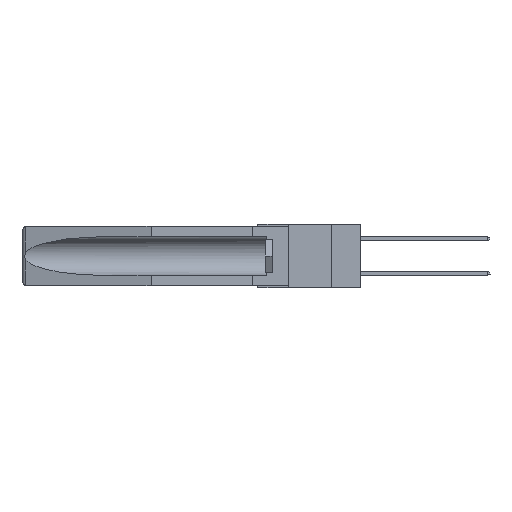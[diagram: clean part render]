
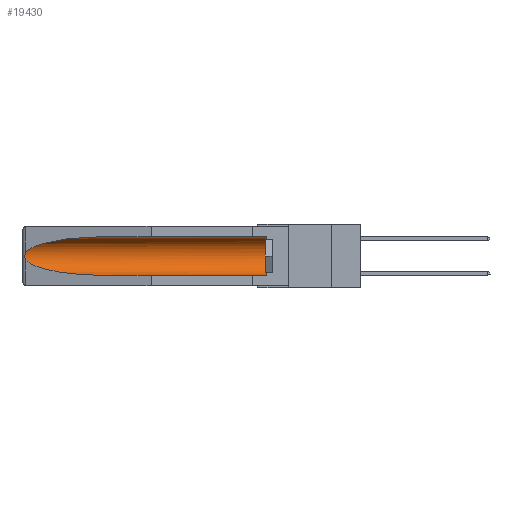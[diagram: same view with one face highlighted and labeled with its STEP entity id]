
A CAD part, left-side view. The second image highlights one B-rep face of the part: STEP entity #19430.
In plain terms, the highlighted cylindrical face has radius 2.857 mm (diameter 5.715 mm), a partial arc.
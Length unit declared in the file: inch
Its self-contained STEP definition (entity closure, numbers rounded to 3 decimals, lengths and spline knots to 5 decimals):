
#130 = CARTESIAN_POINT ( 'NONE',  ( 0.25451, 1.48313, -0.24835 ) ) ;
#312 = EDGE_LOOP ( 'NONE', ( #9508, #18274, #1565, #18513, #764, #6808 ) ) ;
#373 = CARTESIAN_POINT ( 'NONE',  ( 0.2673, 1.53269, -0.17917 ) ) ;
#441 = CARTESIAN_POINT ( 'NONE',  ( 0.2675, 1.53308, -0.16763 ) ) ;
#499 = DIRECTION ( 'NONE',  ( 0., 1., 0. ) ) ;
#579 = EDGE_CURVE ( 'NONE', #10591, #4439, #4516, .T. ) ;
#764 = ORIENTED_EDGE ( 'NONE', *, *, #3685, .T. ) ;
#1401 = CARTESIAN_POINT ( 'NONE',  ( 0.26537, 1.52718, -0.14972 ) ) ;
#1555 = CARTESIAN_POINT ( 'NONE',  ( 0.21114, 1.30732, -0.059 ) ) ;
#1565 = ORIENTED_EDGE ( 'NONE', *, *, #3942, .T. ) ;
#1609 = CARTESIAN_POINT ( 'NONE',  ( 0.21114, 1.30732, -0.284 ) ) ;
#2136 = CARTESIAN_POINT ( 'NONE',  ( 0.26597, 1.5296, -0.19026 ) ) ;
#2745 = DIRECTION ( 'NONE',  ( 0., 0., 1. ) ) ;
#3204 =( BOUNDED_CURVE ( )  B_SPLINE_CURVE ( 3, ( #21183, #1555, #11333, #11249 ),
 .UNSPECIFIED., .F., .F. ) 
 B_SPLINE_CURVE_WITH_KNOTS ( ( 4, 4 ),
 ( 4.71239, 6.08839 ),
 .UNSPECIFIED. ) 
 CURVE ( )  GEOMETRIC_REPRESENTATION_ITEM ( )  RATIONAL_B_SPLINE_CURVE ( ( 1., 0.848, 0.848, 1. ) ) 
 REPRESENTATION_ITEM ( '' )  );
#3685 = EDGE_CURVE ( 'NONE', #10591, #5957, #14403, .T. ) ;
#3721 = EDGE_CURVE ( 'NONE', #5957, #11192, #7472, .T. ) ;
#3915 = B_SPLINE_CURVE_WITH_KNOTS ( 'NONE', 3,
 ( #11846, #15099, #11992, #5355, #441, #16860, #373, #6853, #2136, #18375 ),
 .UNSPECIFIED., .F., .F.,
 ( 4, 2, 2, 2, 4 ),
 ( 0., 0.00029, 0.00058, 0.00087, 0.00117 ),
 .UNSPECIFIED. ) ;
#3942 = EDGE_CURVE ( 'NONE', #12781, #4439, #20276, .T. ) ;
#4372 = CARTESIAN_POINT ( 'NONE',  ( 0.155, 0.126, -0.1715 ) ) ;
#4439 = VERTEX_POINT ( 'NONE', #10927 ) ;
#4516 = LINE ( 'NONE', #18775, #8642 ) ;
#5187 = VECTOR ( 'NONE', #17523, 39.37008 ) ;
#5355 = CARTESIAN_POINT ( 'NONE',  ( 0.2673, 1.5327, -0.16383 ) ) ;
#5412 = EDGE_CURVE ( 'NONE', #11192, #10758, #3204, .T. ) ;
#5437 = AXIS2_PLACEMENT_3D ( 'NONE', #4372, #14287, #2745 ) ;
#5957 = VERTEX_POINT ( 'NONE', #11617 ) ;
#6018 = CARTESIAN_POINT ( 'NONE',  ( 0.155, -0.30754, -0.059 ) ) ;
#6297 = AXIS2_PLACEMENT_3D ( 'NONE', #7346, #13850, #15654 ) ;
#6808 = ORIENTED_EDGE ( 'NONE', *, *, #3721, .T. ) ;
#6853 = CARTESIAN_POINT ( 'NONE',  ( 0.26655, 1.53094, -0.18657 ) ) ;
#7346 = CARTESIAN_POINT ( 'NONE',  ( 0.155, -0.30754, -0.1715 ) ) ;
#7472 = LINE ( 'NONE', #6018, #5187 ) ;
#8642 = VECTOR ( 'NONE', #499, 39.37008 ) ;
#9508 = ORIENTED_EDGE ( 'NONE', *, *, #5412, .T. ) ;
#10166 = FACE_OUTER_BOUND ( 'NONE', #312, .T. ) ;
#10591 = VERTEX_POINT ( 'NONE', #14717 ) ;
#10758 = VERTEX_POINT ( 'NONE', #1401 ) ;
#10927 = CARTESIAN_POINT ( 'NONE',  ( 0.155, 1.07973, -0.284 ) ) ;
#11192 = VERTEX_POINT ( 'NONE', #16958 ) ;
#11226 = CARTESIAN_POINT ( 'NONE',  ( 0.26537, 1.52718, -0.19328 ) ) ;
#11249 = CARTESIAN_POINT ( 'NONE',  ( 0.26537, 1.52718, -0.14972 ) ) ;
#11333 = CARTESIAN_POINT ( 'NONE',  ( 0.25451, 1.48313, -0.09465 ) ) ;
#11617 = CARTESIAN_POINT ( 'NONE',  ( 0.155, 0.126, -0.059 ) ) ;
#11846 = CARTESIAN_POINT ( 'NONE',  ( 0.26537, 1.52718, -0.14972 ) ) ;
#11992 = CARTESIAN_POINT ( 'NONE',  ( 0.26654, 1.53092, -0.15636 ) ) ;
#12337 = EDGE_CURVE ( 'NONE', #10758, #12781, #3915, .T. ) ;
#12781 = VERTEX_POINT ( 'NONE', #20730 ) ;
#13850 = DIRECTION ( 'NONE',  ( 0., 1., 0. ) ) ;
#14287 = DIRECTION ( 'NONE',  ( 0., -1., 0. ) ) ;
#14403 = CIRCLE ( 'NONE', #5437, 0.1125 ) ;
#14717 = CARTESIAN_POINT ( 'NONE',  ( 0.155, 0.126, -0.284 ) ) ;
#15071 = CYLINDRICAL_SURFACE ( 'NONE', #6297, 0.1125 ) ;
#15099 = CARTESIAN_POINT ( 'NONE',  ( 0.26597, 1.52961, -0.15275 ) ) ;
#15654 = DIRECTION ( 'NONE',  ( 0., 0., 1. ) ) ;
#16860 = CARTESIAN_POINT ( 'NONE',  ( 0.2675, 1.53308, -0.17534 ) ) ;
#16958 = CARTESIAN_POINT ( 'NONE',  ( 0.155, 1.07973, -0.059 ) ) ;
#17523 = DIRECTION ( 'NONE',  ( 0., 1., 0. ) ) ;
#18274 = ORIENTED_EDGE ( 'NONE', *, *, #12337, .T. ) ;
#18375 = CARTESIAN_POINT ( 'NONE',  ( 0.26537, 1.52718, -0.19328 ) ) ;
#18513 = ORIENTED_EDGE ( 'NONE', *, *, #579, .F. ) ;
#18775 = CARTESIAN_POINT ( 'NONE',  ( 0.155, -0.30754, -0.284 ) ) ;
#19430 = ADVANCED_FACE ( 'NONE', ( #10166 ), #15071, .F. ) ;
#19872 = CARTESIAN_POINT ( 'NONE',  ( 0.155, 1.07973, -0.284 ) ) ;
#20276 =( BOUNDED_CURVE ( )  B_SPLINE_CURVE ( 3, ( #11226, #130, #1609, #19872 ),
 .UNSPECIFIED., .F., .F. ) 
 B_SPLINE_CURVE_WITH_KNOTS ( ( 4, 4 ),
 ( 0.1948, 1.5708 ),
 .UNSPECIFIED. ) 
 CURVE ( )  GEOMETRIC_REPRESENTATION_ITEM ( )  RATIONAL_B_SPLINE_CURVE ( ( 1., 0.848, 0.848, 1. ) ) 
 REPRESENTATION_ITEM ( '' )  );
#20730 = CARTESIAN_POINT ( 'NONE',  ( 0.26537, 1.52718, -0.19328 ) ) ;
#21183 = CARTESIAN_POINT ( 'NONE',  ( 0.155, 1.07973, -0.059 ) ) ;
